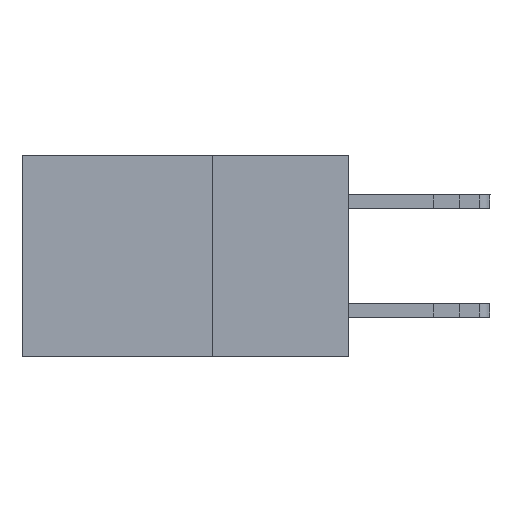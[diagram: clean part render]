
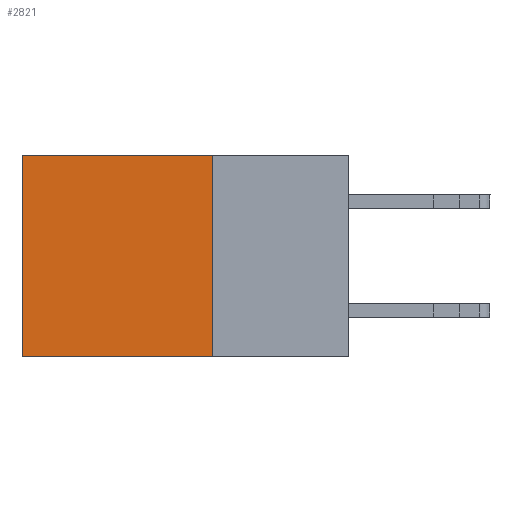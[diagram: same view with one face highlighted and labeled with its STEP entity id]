
A CAD part, left-side view. The second image highlights one B-rep face of the part: STEP entity #2821.
In plain terms, the highlighted planar face has unit normal (-1, 0, 0).
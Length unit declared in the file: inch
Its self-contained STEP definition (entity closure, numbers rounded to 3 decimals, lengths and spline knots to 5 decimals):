
#1838 = DIRECTION ( 'NONE',  ( 0., 0., -1. ) ) ;
#1909 = CARTESIAN_POINT ( 'NONE',  ( 0.298, 0.25, 0. ) ) ;
#2108 = EDGE_CURVE ( 'NONE', #14450, #12602, #22917, .T. ) ;
#2821 = ADVANCED_FACE ( 'NONE', ( #19187 ), #8456, .F. ) ;
#3368 = CARTESIAN_POINT ( 'NONE',  ( 0.298, 0.6, 0. ) ) ;
#4877 = ORIENTED_EDGE ( 'NONE', *, *, #2108, .T. ) ;
#5788 = AXIS2_PLACEMENT_3D ( 'NONE', #21155, #15241, #1838 ) ;
#8456 = PLANE ( 'NONE',  #5788 ) ;
#9416 = ORIENTED_EDGE ( 'NONE', *, *, #10100, .F. ) ;
#9893 = CARTESIAN_POINT ( 'NONE',  ( 0.298, 0.6, -0.37 ) ) ;
#9974 = ORIENTED_EDGE ( 'NONE', *, *, #15388, .T. ) ;
#10100 = EDGE_CURVE ( 'NONE', #10571, #12602, #13359, .T. ) ;
#10571 = VERTEX_POINT ( 'NONE', #13187 ) ;
#12602 = VERTEX_POINT ( 'NONE', #9893 ) ;
#12789 = VECTOR ( 'NONE', #13876, 39.37008 ) ;
#13187 = CARTESIAN_POINT ( 'NONE',  ( 0.298, 0.25, -0.37 ) ) ;
#13359 = LINE ( 'NONE', #19971, #20798 ) ;
#13876 = DIRECTION ( 'NONE',  ( 0., 1., 0. ) ) ;
#14034 = DIRECTION ( 'NONE',  ( 0., 0., -1. ) ) ;
#14285 = ORIENTED_EDGE ( 'NONE', *, *, #18084, .F. ) ;
#14450 = VERTEX_POINT ( 'NONE', #3368 ) ;
#15241 = DIRECTION ( 'NONE',  ( 1., 0., 0. ) ) ;
#15388 = EDGE_CURVE ( 'NONE', #23343, #14450, #18120, .T. ) ;
#18006 = EDGE_LOOP ( 'NONE', ( #4877, #9416, #14285, #9974 ) ) ;
#18011 = VECTOR ( 'NONE', #18541, 39.37008 ) ;
#18084 = EDGE_CURVE ( 'NONE', #23343, #10571, #24742, .T. ) ;
#18120 = LINE ( 'NONE', #26872, #12789 ) ;
#18541 = DIRECTION ( 'NONE',  ( 0., 0., -1. ) ) ;
#19187 = FACE_OUTER_BOUND ( 'NONE', #18006, .T. ) ;
#19971 = CARTESIAN_POINT ( 'NONE',  ( 0.298, 0.25, -0.37 ) ) ;
#20238 = CARTESIAN_POINT ( 'NONE',  ( 0.298, 0.25, 0. ) ) ;
#20798 = VECTOR ( 'NONE', #21947, 39.37008 ) ;
#21155 = CARTESIAN_POINT ( 'NONE',  ( 0.298, 0.25, 0. ) ) ;
#21901 = VECTOR ( 'NONE', #14034, 39.37008 ) ;
#21947 = DIRECTION ( 'NONE',  ( 0., 1., 0. ) ) ;
#22917 = LINE ( 'NONE', #24898, #18011 ) ;
#23343 = VERTEX_POINT ( 'NONE', #1909 ) ;
#24742 = LINE ( 'NONE', #20238, #21901 ) ;
#24898 = CARTESIAN_POINT ( 'NONE',  ( 0.298, 0.6, 0. ) ) ;
#26872 = CARTESIAN_POINT ( 'NONE',  ( 0.298, 0.25, 0. ) ) ;
